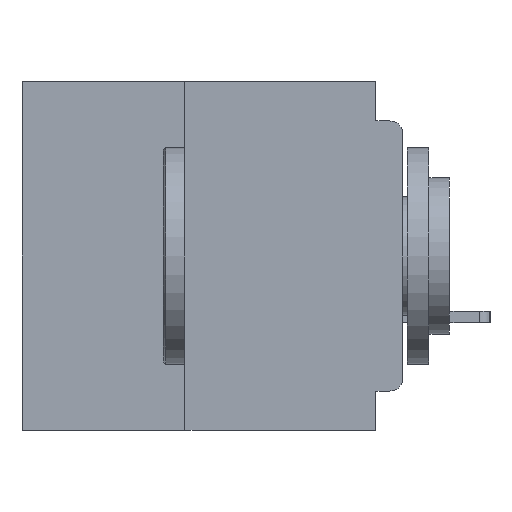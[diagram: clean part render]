
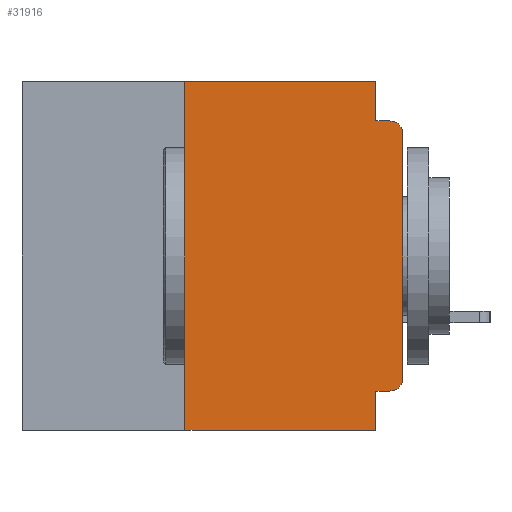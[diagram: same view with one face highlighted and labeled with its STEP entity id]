
A CAD part, left-side view. The second image highlights one B-rep face of the part: STEP entity #31916.
In plain terms, the highlighted planar face has unit normal (-1, 0, 0).
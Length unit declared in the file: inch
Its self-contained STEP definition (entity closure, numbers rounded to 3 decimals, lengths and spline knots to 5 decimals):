
#82 = VERTEX_POINT ( 'NONE', #11303 ) ;
#498 = VERTEX_POINT ( 'NONE', #27413 ) ;
#618 = EDGE_CURVE ( 'NONE', #498, #27758, #41164, .T. ) ;
#2331 = LINE ( 'NONE', #11353, #11828 ) ;
#3138 = VERTEX_POINT ( 'NONE', #4746 ) ;
#3302 = CARTESIAN_POINT ( 'NONE',  ( 0., 0.015, -0.06 ) ) ;
#3316 = EDGE_CURVE ( 'NONE', #35258, #24697, #31675, .T. ) ;
#3396 = EDGE_LOOP ( 'NONE', ( #6109, #11527, #7483, #20206, #36333, #6141, #3786, #40902, #9836, #11901 ) ) ;
#3426 = VERTEX_POINT ( 'NONE', #6561 ) ;
#3758 = CARTESIAN_POINT ( 'NONE',  ( 0., 0.031, 0. ) ) ;
#3786 = ORIENTED_EDGE ( 'NONE', *, *, #27788, .T. ) ;
#4042 = PLANE ( 'NONE',  #17851 ) ;
#4066 = DIRECTION ( 'NONE',  ( 0., 0., 1. ) ) ;
#4746 = CARTESIAN_POINT ( 'NONE',  ( 0., 0.031, -0.045 ) ) ;
#6109 = ORIENTED_EDGE ( 'NONE', *, *, #18825, .T. ) ;
#6141 = ORIENTED_EDGE ( 'NONE', *, *, #17227, .F. ) ;
#6561 = CARTESIAN_POINT ( 'NONE',  ( 0., 0.25, -0.4 ) ) ;
#6588 = AXIS2_PLACEMENT_3D ( 'NONE', #3302, #27805, #6968 ) ;
#6968 = DIRECTION ( 'NONE',  ( 0., 0., -1. ) ) ;
#7483 = ORIENTED_EDGE ( 'NONE', *, *, #41554, .F. ) ;
#8571 = LINE ( 'NONE', #39181, #25958 ) ;
#9836 = ORIENTED_EDGE ( 'NONE', *, *, #34797, .F. ) ;
#10235 = CARTESIAN_POINT ( 'NONE',  ( 0., 0.031, -0.4 ) ) ;
#10367 = DIRECTION ( 'NONE',  ( 0., 1., 0. ) ) ;
#11231 = DIRECTION ( 'NONE',  ( 1., 0., 0. ) ) ;
#11303 = CARTESIAN_POINT ( 'NONE',  ( 0., 0., -0.06 ) ) ;
#11353 = CARTESIAN_POINT ( 'NONE',  ( 0., 0., -0.045 ) ) ;
#11527 = ORIENTED_EDGE ( 'NONE', *, *, #17556, .T. ) ;
#11828 = VECTOR ( 'NONE', #21806, 39.37008 ) ;
#11901 = ORIENTED_EDGE ( 'NONE', *, *, #3316, .T. ) ;
#15350 = FACE_OUTER_BOUND ( 'NONE', #3396, .T. ) ;
#15449 = VERTEX_POINT ( 'NONE', #3758 ) ;
#17227 = EDGE_CURVE ( 'NONE', #3426, #38395, #23812, .T. ) ;
#17556 = EDGE_CURVE ( 'NONE', #82, #39335, #30279, .T. ) ;
#17681 = CARTESIAN_POINT ( 'NONE',  ( 0., 0., 0. ) ) ;
#17846 = DIRECTION ( 'NONE',  ( 0., -1., 0. ) ) ;
#17851 = AXIS2_PLACEMENT_3D ( 'NONE', #24879, #11231, #35501 ) ;
#18762 = LINE ( 'NONE', #17681, #36143 ) ;
#18825 = EDGE_CURVE ( 'NONE', #24697, #82, #18762, .T. ) ;
#19097 = EDGE_CURVE ( 'NONE', #38395, #15449, #25242, .T. ) ;
#20007 = DIRECTION ( 'NONE',  ( -1., 0., 0. ) ) ;
#20206 = ORIENTED_EDGE ( 'NONE', *, *, #26141, .F. ) ;
#21806 = DIRECTION ( 'NONE',  ( 0., -1., 0. ) ) ;
#23812 = LINE ( 'NONE', #38848, #41168 ) ;
#24653 = DIRECTION ( 'NONE',  ( 0., 0., 1. ) ) ;
#24697 = VERTEX_POINT ( 'NONE', #43320 ) ;
#24879 = CARTESIAN_POINT ( 'NONE',  ( 0., 0.437, 0. ) ) ;
#25242 = LINE ( 'NONE', #43464, #42625 ) ;
#25958 = VECTOR ( 'NONE', #42714, 39.37008 ) ;
#26062 = LINE ( 'NONE', #38735, #34206 ) ;
#26141 = EDGE_CURVE ( 'NONE', #15449, #3138, #8571, .T. ) ;
#26153 = DIRECTION ( 'NONE',  ( 0., -1., 0. ) ) ;
#27413 = CARTESIAN_POINT ( 'NONE',  ( 0., 0.031, -0.355 ) ) ;
#27758 = VERTEX_POINT ( 'NONE', #34978 ) ;
#27788 = EDGE_CURVE ( 'NONE', #3426, #27758, #30131, .T. ) ;
#27805 = DIRECTION ( 'NONE',  ( -1., 0., 0. ) ) ;
#29852 = CARTESIAN_POINT ( 'NONE',  ( 0., 0.25, 0. ) ) ;
#30131 = LINE ( 'NONE', #42120, #39342 ) ;
#30279 = CIRCLE ( 'NONE', #6588, 0.015 ) ;
#31675 = CIRCLE ( 'NONE', #34070, 0.015 ) ;
#31916 = ADVANCED_FACE ( 'NONE', ( #15350 ), #4042, .F. ) ;
#31931 = VECTOR ( 'NONE', #33500, 39.37008 ) ;
#33500 = DIRECTION ( 'NONE',  ( 0., 0., -1. ) ) ;
#34070 = AXIS2_PLACEMENT_3D ( 'NONE', #40775, #20007, #44282 ) ;
#34206 = VECTOR ( 'NONE', #10367, 39.37008 ) ;
#34797 = EDGE_CURVE ( 'NONE', #35258, #498, #26062, .T. ) ;
#34978 = CARTESIAN_POINT ( 'NONE',  ( 0., 0.031, -0.4 ) ) ;
#35258 = VERTEX_POINT ( 'NONE', #37653 ) ;
#35501 = DIRECTION ( 'NONE',  ( 0., 0., -1. ) ) ;
#36143 = VECTOR ( 'NONE', #24653, 39.37008 ) ;
#36333 = ORIENTED_EDGE ( 'NONE', *, *, #19097, .F. ) ;
#37653 = CARTESIAN_POINT ( 'NONE',  ( 0., 0.015, -0.355 ) ) ;
#38395 = VERTEX_POINT ( 'NONE', #29852 ) ;
#38735 = CARTESIAN_POINT ( 'NONE',  ( 0., 0., -0.355 ) ) ;
#38848 = CARTESIAN_POINT ( 'NONE',  ( 0., 0.25, -0.4 ) ) ;
#38864 = CARTESIAN_POINT ( 'NONE',  ( 0., 0.015, -0.045 ) ) ;
#39181 = CARTESIAN_POINT ( 'NONE',  ( 0., 0.031, 0. ) ) ;
#39335 = VERTEX_POINT ( 'NONE', #38864 ) ;
#39342 = VECTOR ( 'NONE', #17846, 39.37008 ) ;
#40775 = CARTESIAN_POINT ( 'NONE',  ( 0., 0.015, -0.34 ) ) ;
#40902 = ORIENTED_EDGE ( 'NONE', *, *, #618, .F. ) ;
#41164 = LINE ( 'NONE', #10235, #31931 ) ;
#41168 = VECTOR ( 'NONE', #4066, 39.37008 ) ;
#41554 = EDGE_CURVE ( 'NONE', #3138, #39335, #2331, .T. ) ;
#42120 = CARTESIAN_POINT ( 'NONE',  ( 0., 0.437, -0.4 ) ) ;
#42625 = VECTOR ( 'NONE', #26153, 39.37008 ) ;
#42714 = DIRECTION ( 'NONE',  ( 0., 0., -1. ) ) ;
#43320 = CARTESIAN_POINT ( 'NONE',  ( 0., 0., -0.34 ) ) ;
#43464 = CARTESIAN_POINT ( 'NONE',  ( 0., 0.437, 0. ) ) ;
#44282 = DIRECTION ( 'NONE',  ( 0., 0., -1. ) ) ;
